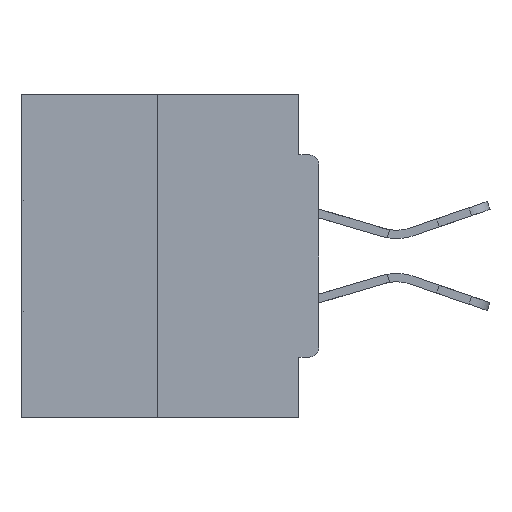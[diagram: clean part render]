
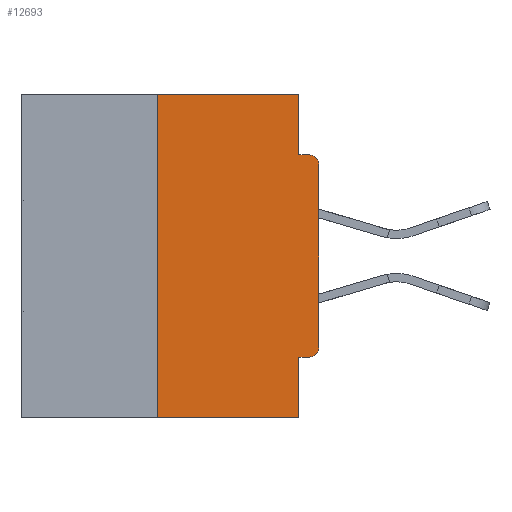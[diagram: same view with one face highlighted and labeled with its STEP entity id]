
A CAD part, left-side view. The second image highlights one B-rep face of the part: STEP entity #12693.
In plain terms, the highlighted planar face has unit normal (-1, 0, 0).
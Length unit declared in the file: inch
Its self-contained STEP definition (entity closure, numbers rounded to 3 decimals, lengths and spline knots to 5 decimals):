
#313 = ORIENTED_EDGE ( 'NONE', *, *, #36045, .F. ) ;
#546 = CARTESIAN_POINT ( 'NONE',  ( 0., 0., 0. ) ) ;
#741 = CARTESIAN_POINT ( 'NONE',  ( 0., 0.015, -0.0935 ) ) ;
#766 = VECTOR ( 'NONE', #9843, 39.37008 ) ;
#930 = ORIENTED_EDGE ( 'NONE', *, *, #30106, .T. ) ;
#935 = CARTESIAN_POINT ( 'NONE',  ( 0., 0.46, 0. ) ) ;
#1050 = VERTEX_POINT ( 'NONE', #24289 ) ;
#1199 = VECTOR ( 'NONE', #31740, 39.37008 ) ;
#1474 = DIRECTION ( 'NONE',  ( 0., 0., 1. ) ) ;
#2295 = VERTEX_POINT ( 'NONE', #39593 ) ;
#2619 = PLANE ( 'NONE',  #15971 ) ;
#2640 = CARTESIAN_POINT ( 'NONE',  ( 0., 0.46, -0.5 ) ) ;
#2973 = AXIS2_PLACEMENT_3D ( 'NONE', #37380, #33748, #12054 ) ;
#3439 = EDGE_CURVE ( 'NONE', #34155, #6464, #26663, .T. ) ;
#3573 = CARTESIAN_POINT ( 'NONE',  ( 0., 0., -0.0935 ) ) ;
#3659 = DIRECTION ( 'NONE',  ( 0., 0., 1. ) ) ;
#3828 = VERTEX_POINT ( 'NONE', #741 ) ;
#5015 = EDGE_CURVE ( 'NONE', #32211, #15984, #39675, .T. ) ;
#5063 = ORIENTED_EDGE ( 'NONE', *, *, #28361, .F. ) ;
#5116 = ORIENTED_EDGE ( 'NONE', *, *, #3439, .F. ) ;
#5510 = DIRECTION ( 'NONE',  ( 0., -1., 0. ) ) ;
#6455 = CARTESIAN_POINT ( 'NONE',  ( 0., 0., -0.3915 ) ) ;
#6464 = VERTEX_POINT ( 'NONE', #29278 ) ;
#6704 = DIRECTION ( 'NONE',  ( 0., -1., 0. ) ) ;
#8561 = EDGE_CURVE ( 'NONE', #1050, #2295, #17286, .T. ) ;
#8636 = ORIENTED_EDGE ( 'NONE', *, *, #39868, .F. ) ;
#9056 = VECTOR ( 'NONE', #1474, 39.37008 ) ;
#9843 = DIRECTION ( 'NONE',  ( 0., 0., -1. ) ) ;
#10649 = EDGE_CURVE ( 'NONE', #34155, #28867, #17133, .T. ) ;
#10910 = EDGE_LOOP ( 'NONE', ( #10957, #5116, #11510, #5063, #313, #32791, #38806, #930, #8636, #36853 ) ) ;
#10957 = ORIENTED_EDGE ( 'NONE', *, *, #13797, .F. ) ;
#11344 = DIRECTION ( 'NONE',  ( 0., 0., -1. ) ) ;
#11472 = CARTESIAN_POINT ( 'NONE',  ( 0., 0.46, 0. ) ) ;
#11510 = ORIENTED_EDGE ( 'NONE', *, *, #10649, .T. ) ;
#12054 = DIRECTION ( 'NONE',  ( 0., 0., -1. ) ) ;
#12500 = LINE ( 'NONE', #935, #29582 ) ;
#12693 = ADVANCED_FACE ( 'NONE', ( #20461 ), #2619, .F. ) ;
#12828 = CARTESIAN_POINT ( 'NONE',  ( 0., 0.031, 0. ) ) ;
#13326 = VERTEX_POINT ( 'NONE', #24490 ) ;
#13797 = EDGE_CURVE ( 'NONE', #6464, #1050, #12500, .T. ) ;
#14660 = CIRCLE ( 'NONE', #2973, 0.015 ) ;
#15293 = CARTESIAN_POINT ( 'NONE',  ( 0., 0.015, -0.3915 ) ) ;
#15971 = AXIS2_PLACEMENT_3D ( 'NONE', #11472, #30397, #11344 ) ;
#15984 = VERTEX_POINT ( 'NONE', #18595 ) ;
#16151 = CARTESIAN_POINT ( 'NONE',  ( 0., 0.031, -0.5 ) ) ;
#16606 = CARTESIAN_POINT ( 'NONE',  ( 0., 0.25, -0.5 ) ) ;
#17075 = CARTESIAN_POINT ( 'NONE',  ( 0., 0.25, 0. ) ) ;
#17133 = LINE ( 'NONE', #2640, #25948 ) ;
#17286 = LINE ( 'NONE', #12828, #766 ) ;
#18595 = CARTESIAN_POINT ( 'NONE',  ( 0., 0., -0.1085 ) ) ;
#19892 = VECTOR ( 'NONE', #26024, 39.37008 ) ;
#20461 = FACE_OUTER_BOUND ( 'NONE', #10910, .T. ) ;
#21569 = DIRECTION ( 'NONE',  ( 0., 0., -1. ) ) ;
#23753 = VERTEX_POINT ( 'NONE', #27973 ) ;
#24289 = CARTESIAN_POINT ( 'NONE',  ( 0., 0.031, 0. ) ) ;
#24490 = CARTESIAN_POINT ( 'NONE',  ( 0., 0.015, -0.4065 ) ) ;
#25948 = VECTOR ( 'NONE', #5510, 39.37008 ) ;
#26024 = DIRECTION ( 'NONE',  ( 0., 1., 0. ) ) ;
#26663 = LINE ( 'NONE', #17075, #9056 ) ;
#27973 = CARTESIAN_POINT ( 'NONE',  ( 0., 0.031, -0.4065 ) ) ;
#28361 = EDGE_CURVE ( 'NONE', #23753, #28867, #33855, .T. ) ;
#28867 = VERTEX_POINT ( 'NONE', #33030 ) ;
#29083 = LINE ( 'NONE', #3573, #32026 ) ;
#29275 = CARTESIAN_POINT ( 'NONE',  ( 0., 0., -0.4065 ) ) ;
#29278 = CARTESIAN_POINT ( 'NONE',  ( 0., 0.25, 0. ) ) ;
#29582 = VECTOR ( 'NONE', #38470, 39.37008 ) ;
#30106 = EDGE_CURVE ( 'NONE', #15984, #3828, #14660, .T. ) ;
#30175 = EDGE_CURVE ( 'NONE', #13326, #32211, #31250, .T. ) ;
#30397 = DIRECTION ( 'NONE',  ( 1., 0., 0. ) ) ;
#31250 = CIRCLE ( 'NONE', #35748, 0.015 ) ;
#31740 = DIRECTION ( 'NONE',  ( 0., 0., -1. ) ) ;
#32026 = VECTOR ( 'NONE', #6704, 39.37008 ) ;
#32211 = VERTEX_POINT ( 'NONE', #6455 ) ;
#32386 = VECTOR ( 'NONE', #3659, 39.37008 ) ;
#32791 = ORIENTED_EDGE ( 'NONE', *, *, #30175, .T. ) ;
#33030 = CARTESIAN_POINT ( 'NONE',  ( 0., 0.031, -0.5 ) ) ;
#33748 = DIRECTION ( 'NONE',  ( -1., 0., 0. ) ) ;
#33855 = LINE ( 'NONE', #16151, #1199 ) ;
#34155 = VERTEX_POINT ( 'NONE', #16606 ) ;
#35748 = AXIS2_PLACEMENT_3D ( 'NONE', #15293, #40255, #21569 ) ;
#36045 = EDGE_CURVE ( 'NONE', #13326, #23753, #37895, .T. ) ;
#36853 = ORIENTED_EDGE ( 'NONE', *, *, #8561, .F. ) ;
#37380 = CARTESIAN_POINT ( 'NONE',  ( 0., 0.015, -0.1085 ) ) ;
#37895 = LINE ( 'NONE', #29275, #19892 ) ;
#38470 = DIRECTION ( 'NONE',  ( 0., -1., 0. ) ) ;
#38806 = ORIENTED_EDGE ( 'NONE', *, *, #5015, .T. ) ;
#39593 = CARTESIAN_POINT ( 'NONE',  ( 0., 0.031, -0.0935 ) ) ;
#39675 = LINE ( 'NONE', #546, #32386 ) ;
#39868 = EDGE_CURVE ( 'NONE', #2295, #3828, #29083, .T. ) ;
#40255 = DIRECTION ( 'NONE',  ( -1., 0., 0. ) ) ;
